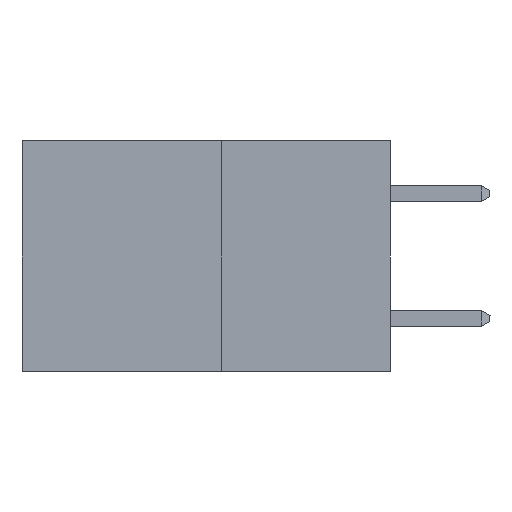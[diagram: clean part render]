
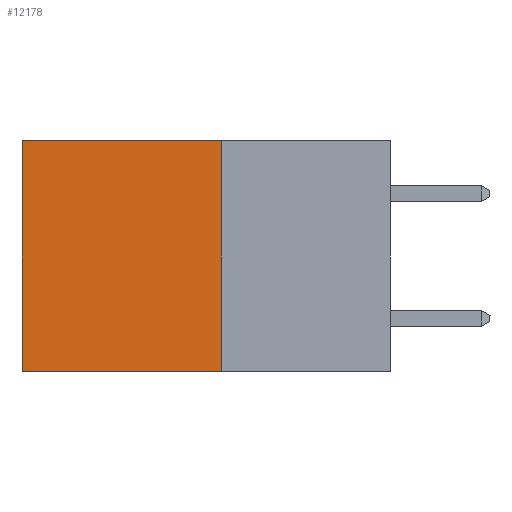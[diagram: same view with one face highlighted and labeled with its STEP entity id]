
A CAD part, left-side view. The second image highlights one B-rep face of the part: STEP entity #12178.
In plain terms, the highlighted planar face has unit normal (-1, 0, 0).
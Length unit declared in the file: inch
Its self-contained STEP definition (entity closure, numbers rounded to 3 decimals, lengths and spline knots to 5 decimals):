
#104 = DIRECTION ( 'NONE',  ( 0., 0., -1. ) ) ;
#1703 = CARTESIAN_POINT ( 'NONE',  ( 0.277, 0.27, -0.37 ) ) ;
#1831 = ORIENTED_EDGE ( 'NONE', *, *, #19139, .T. ) ;
#2618 = CARTESIAN_POINT ( 'NONE',  ( 0.277, 0.59, -0.37 ) ) ;
#2795 = VECTOR ( 'NONE', #26597, 39.37008 ) ;
#3638 = CARTESIAN_POINT ( 'NONE',  ( 0.277, 0.27, 0. ) ) ;
#3656 = LINE ( 'NONE', #3638, #2795 ) ;
#4361 = DIRECTION ( 'NONE',  ( 0., 1., 0. ) ) ;
#7972 = VERTEX_POINT ( 'NONE', #20455 ) ;
#9063 = VECTOR ( 'NONE', #104, 39.37008 ) ;
#9100 = DIRECTION ( 'NONE',  ( 0., 0., -1. ) ) ;
#9972 = VECTOR ( 'NONE', #9100, 39.37008 ) ;
#10994 = PLANE ( 'NONE',  #13015 ) ;
#12178 = ADVANCED_FACE ( 'NONE', ( #25861 ), #10994, .F. ) ;
#12965 = LINE ( 'NONE', #1703, #18172 ) ;
#13015 = AXIS2_PLACEMENT_3D ( 'NONE', #28849, #31397, #16085 ) ;
#15278 = EDGE_CURVE ( 'NONE', #17900, #7972, #21773, .T. ) ;
#15789 = ORIENTED_EDGE ( 'NONE', *, *, #22729, .T. ) ;
#15816 = VERTEX_POINT ( 'NONE', #2618 ) ;
#16085 = DIRECTION ( 'NONE',  ( 0., 0., -1. ) ) ;
#16640 = ORIENTED_EDGE ( 'NONE', *, *, #15278, .F. ) ;
#17339 = CARTESIAN_POINT ( 'NONE',  ( 0.277, 0.27, 0. ) ) ;
#17900 = VERTEX_POINT ( 'NONE', #17339 ) ;
#18172 = VECTOR ( 'NONE', #4361, 39.37008 ) ;
#19139 = EDGE_CURVE ( 'NONE', #25873, #15816, #23520, .T. ) ;
#20455 = CARTESIAN_POINT ( 'NONE',  ( 0.277, 0.27, -0.37 ) ) ;
#21773 = LINE ( 'NONE', #30907, #9063 ) ;
#22729 = EDGE_CURVE ( 'NONE', #17900, #25873, #3656, .T. ) ;
#23520 = LINE ( 'NONE', #26904, #9972 ) ;
#23525 = ORIENTED_EDGE ( 'NONE', *, *, #28371, .F. ) ;
#25861 = FACE_OUTER_BOUND ( 'NONE', #28439, .T. ) ;
#25873 = VERTEX_POINT ( 'NONE', #25955 ) ;
#25955 = CARTESIAN_POINT ( 'NONE',  ( 0.277, 0.59, 0. ) ) ;
#26597 = DIRECTION ( 'NONE',  ( 0., 1., 0. ) ) ;
#26904 = CARTESIAN_POINT ( 'NONE',  ( 0.277, 0.59, -0.37 ) ) ;
#28371 = EDGE_CURVE ( 'NONE', #7972, #15816, #12965, .T. ) ;
#28439 = EDGE_LOOP ( 'NONE', ( #1831, #23525, #16640, #15789 ) ) ;
#28849 = CARTESIAN_POINT ( 'NONE',  ( 0.277, 0.27, -0.37 ) ) ;
#30907 = CARTESIAN_POINT ( 'NONE',  ( 0.277, 0.27, -0.37 ) ) ;
#31397 = DIRECTION ( 'NONE',  ( 1., 0., 0. ) ) ;
